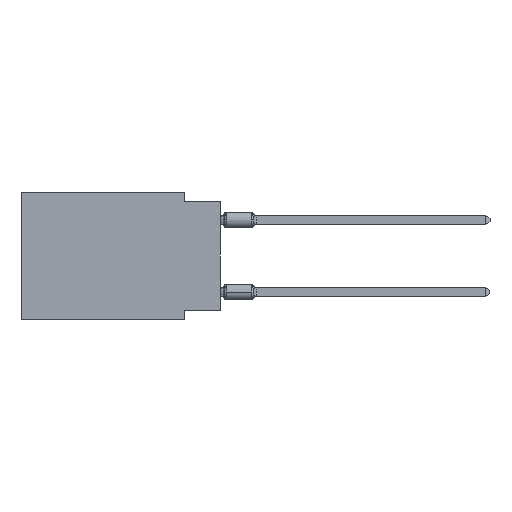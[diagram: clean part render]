
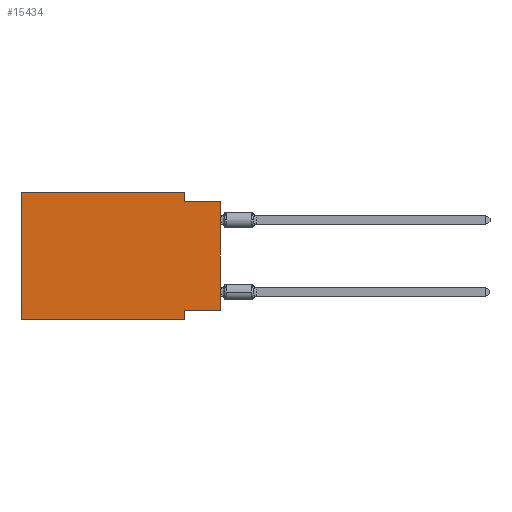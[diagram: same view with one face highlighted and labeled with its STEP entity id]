
A CAD part, left-side view. The second image highlights one B-rep face of the part: STEP entity #15434.
In plain terms, the highlighted planar face has unit normal (-1, 0, 0).
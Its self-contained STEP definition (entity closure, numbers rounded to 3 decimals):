
#122 = EDGE_CURVE ( 'NONE', #8885, #794, #9707, .T. ) ;
#794 = VERTEX_POINT ( 'NONE', #1893 ) ;
#1727 = CARTESIAN_POINT ( 'NONE',  ( 0., 2.54, 0. ) ) ;
#1893 = CARTESIAN_POINT ( 'NONE',  ( 0., 13.97, 0. ) ) ;
#2286 = CARTESIAN_POINT ( 'NONE',  ( 0., 0., -8.255 ) ) ;
#2605 = DIRECTION ( 'NONE',  ( 0., -1., 0. ) ) ;
#3089 = VECTOR ( 'NONE', #16246, 1000. ) ;
#3179 = CARTESIAN_POINT ( 'NONE',  ( 0., 0., -0.635 ) ) ;
#3252 = DIRECTION ( 'NONE',  ( 0., 0., -1. ) ) ;
#3537 = LINE ( 'NONE', #3179, #6060 ) ;
#3800 = EDGE_CURVE ( 'NONE', #8885, #12754, #17214, .T. ) ;
#3948 = DIRECTION ( 'NONE',  ( 0., 0., 1. ) ) ;
#4266 = EDGE_CURVE ( 'NONE', #12302, #6067, #3537, .T. ) ;
#4275 = CARTESIAN_POINT ( 'NONE',  ( 0., 13.97, 0. ) ) ;
#4555 = EDGE_CURVE ( 'NONE', #6452, #6067, #11224, .T. ) ;
#4728 = CARTESIAN_POINT ( 'NONE',  ( 0., 13.97, 0. ) ) ;
#5220 = ORIENTED_EDGE ( 'NONE', *, *, #9536, .F. ) ;
#5264 = CARTESIAN_POINT ( 'NONE',  ( 0., 2.54, -8.89 ) ) ;
#5499 = EDGE_CURVE ( 'NONE', #6452, #15652, #9137, .T. ) ;
#5759 = CARTESIAN_POINT ( 'NONE',  ( 0., 0., 0. ) ) ;
#5857 = DIRECTION ( 'NONE',  ( 1., 0., 0. ) ) ;
#5887 = DIRECTION ( 'NONE',  ( 0., 0., -1. ) ) ;
#5960 = VECTOR ( 'NONE', #2605, 1000. ) ;
#5971 = EDGE_CURVE ( 'NONE', #15652, #12754, #14666, .T. ) ;
#6060 = VECTOR ( 'NONE', #14482, 1000. ) ;
#6067 = VERTEX_POINT ( 'NONE', #15465 ) ;
#6452 = VERTEX_POINT ( 'NONE', #2286 ) ;
#6829 = CARTESIAN_POINT ( 'NONE',  ( 0., 13.97, -8.89 ) ) ;
#7741 = VECTOR ( 'NONE', #3948, 1000. ) ;
#7858 = ORIENTED_EDGE ( 'NONE', *, *, #4555, .T. ) ;
#8259 = LINE ( 'NONE', #4275, #5960 ) ;
#8614 = AXIS2_PLACEMENT_3D ( 'NONE', #4728, #5857, #3252 ) ;
#8733 = ORIENTED_EDGE ( 'NONE', *, *, #3800, .T. ) ;
#8885 = VERTEX_POINT ( 'NONE', #6829 ) ;
#8969 = ORIENTED_EDGE ( 'NONE', *, *, #122, .F. ) ;
#9022 = VECTOR ( 'NONE', #10182, 1000. ) ;
#9137 = LINE ( 'NONE', #12188, #3089 ) ;
#9524 = CARTESIAN_POINT ( 'NONE',  ( 0., 13.97, 0. ) ) ;
#9536 = EDGE_CURVE ( 'NONE', #13581, #12302, #18284, .T. ) ;
#9707 = LINE ( 'NONE', #9524, #7741 ) ;
#9830 = ORIENTED_EDGE ( 'NONE', *, *, #15324, .F. ) ;
#10025 = DIRECTION ( 'NONE',  ( 0., 0., 1. ) ) ;
#10182 = DIRECTION ( 'NONE',  ( 0., -1., 0. ) ) ;
#10272 = ORIENTED_EDGE ( 'NONE', *, *, #5499, .F. ) ;
#11224 = LINE ( 'NONE', #5759, #11362 ) ;
#11362 = VECTOR ( 'NONE', #10025, 1000. ) ;
#12188 = CARTESIAN_POINT ( 'NONE',  ( 0., 0., -8.255 ) ) ;
#12302 = VERTEX_POINT ( 'NONE', #16707 ) ;
#12410 = EDGE_LOOP ( 'NONE', ( #7858, #18229, #5220, #9830, #8969, #8733, #15791, #10272 ) ) ;
#12754 = VERTEX_POINT ( 'NONE', #16784 ) ;
#13581 = VERTEX_POINT ( 'NONE', #1727 ) ;
#13593 = VECTOR ( 'NONE', #5887, 1000. ) ;
#13793 = DIRECTION ( 'NONE',  ( 0., 0., -1. ) ) ;
#14482 = DIRECTION ( 'NONE',  ( 0., -1., 0. ) ) ;
#14529 = CARTESIAN_POINT ( 'NONE',  ( 0., 13.97, -8.89 ) ) ;
#14666 = LINE ( 'NONE', #5264, #16173 ) ;
#15324 = EDGE_CURVE ( 'NONE', #794, #13581, #8259, .T. ) ;
#15434 = ADVANCED_FACE ( 'NONE', ( #15947 ), #15856, .F. ) ;
#15465 = CARTESIAN_POINT ( 'NONE',  ( 0., 0., -0.635 ) ) ;
#15652 = VERTEX_POINT ( 'NONE', #16723 ) ;
#15791 = ORIENTED_EDGE ( 'NONE', *, *, #5971, .F. ) ;
#15856 = PLANE ( 'NONE',  #8614 ) ;
#15947 = FACE_OUTER_BOUND ( 'NONE', #12410, .T. ) ;
#16173 = VECTOR ( 'NONE', #13793, 1000. ) ;
#16246 = DIRECTION ( 'NONE',  ( 0., 1., 0. ) ) ;
#16707 = CARTESIAN_POINT ( 'NONE',  ( 0., 2.54, -0.635 ) ) ;
#16723 = CARTESIAN_POINT ( 'NONE',  ( 0., 2.54, -8.255 ) ) ;
#16784 = CARTESIAN_POINT ( 'NONE',  ( 0., 2.54, -8.89 ) ) ;
#16906 = CARTESIAN_POINT ( 'NONE',  ( 0., 2.54, 0. ) ) ;
#17214 = LINE ( 'NONE', #14529, #9022 ) ;
#18229 = ORIENTED_EDGE ( 'NONE', *, *, #4266, .F. ) ;
#18284 = LINE ( 'NONE', #16906, #13593 ) ;
